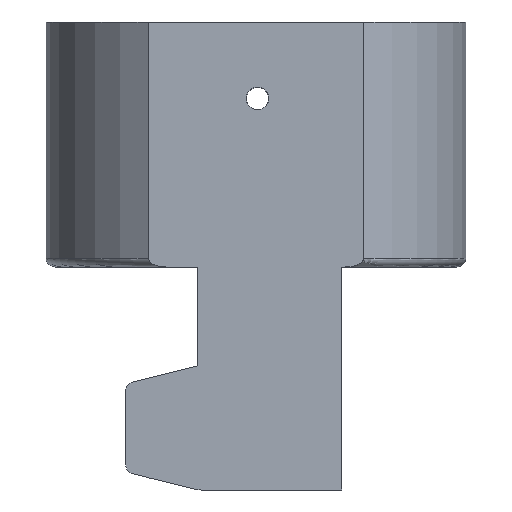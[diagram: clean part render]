
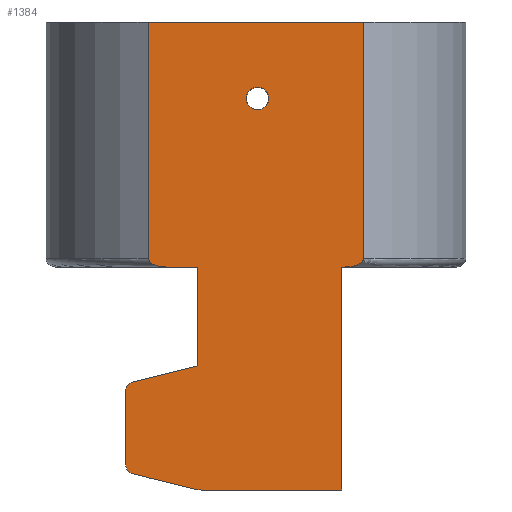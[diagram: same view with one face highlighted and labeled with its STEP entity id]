
A CAD part, front view. The second image highlights one B-rep face of the part: STEP entity #1384.
In plain terms, the highlighted planar face has unit normal (0, -1, 0).
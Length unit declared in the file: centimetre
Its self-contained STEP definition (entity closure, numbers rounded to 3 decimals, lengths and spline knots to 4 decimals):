
#66=FACE_BOUND($,#262,.T.);
#82=PLANE($,#1468);
#96=LINE($,#1725,#133);
#106=LINE($,#1777,#143);
#107=LINE($,#1780,#144);
#109=LINE($,#1786,#146);
#110=LINE($,#1789,#147);
#111=LINE($,#1792,#148);
#114=LINE($,#1802,#151);
#120=LINE($,#1924,#157);
#122=LINE($,#1928,#159);
#123=LINE($,#1932,#160);
#124=LINE($,#1935,#161);
#133=VECTOR($,#1518,2.595);
#143=VECTOR($,#1542,0.339);
#144=VECTOR($,#1545,0.0324);
#146=VECTOR($,#1551,2.3692);
#147=VECTOR($,#1556,2.595);
#148=VECTOR($,#1559,2.4514);
#151=VECTOR($,#1568,1.0861);
#157=VECTOR($,#1604,0.7391);
#159=VECTOR($,#1608,0.8148);
#160=VECTOR($,#1611,0.7025);
#161=VECTOR($,#1614,1.5474);
#199=FACE_OUTER_BOUND($,#261,.T.);
#261=EDGE_LOOP($,(#981,#982,#983,#984,#985,#986,#987,#988,#989,#990,#991,
#992,#993,#994,#995,#996));
#262=EDGE_LOOP($,(#997));
#323=CIRCLE($,#1454,0.099);
#331=CIRCLE($,#1469,0.099);
#332=CIRCLE($,#1470,0.297);
#333=CIRCLE($,#1471,0.1238);
#344=B_SPLINE_CURVE_WITH_KNOTS($,3,(#1707,#1708,#1709,#1710,#1711,#1712,
#1713,#1714,#1715,#1716,#1717,#1718),.UNSPECIFIED.,.F.,.F.,(4,2,2,2,2,4),
(1.0104,1.0239,1.039,1.0807,1.1452,
1.2445),.UNSPECIFIED.);
#346=B_SPLINE_CURVE_WITH_KNOTS($,3,(#1760,#1761,#1762,#1763,#1764,#1765,
#1766,#1767,#1768,#1769,#1770,#1771),.UNSPECIFIED.,.F.,.F.,(4,2,2,2,2,4),
(0.7762,0.8756,0.9401,0.9818,
0.9968,1.0104),.UNSPECIFIED.);
#487=VERTEX_POINT($,#1704);
#488=VERTEX_POINT($,#1706);
#490=VERTEX_POINT($,#1723);
#501=VERTEX_POINT($,#1758);
#502=VERTEX_POINT($,#1759);
#503=VERTEX_POINT($,#1775);
#504=VERTEX_POINT($,#1779);
#506=VERTEX_POINT($,#1785);
#507=VERTEX_POINT($,#1791);
#511=VERTEX_POINT($,#1801);
#512=VERTEX_POINT($,#1805);
#513=VERTEX_POINT($,#1806);
#525=VERTEX_POINT($,#1927);
#526=VERTEX_POINT($,#1929);
#527=VERTEX_POINT($,#1931);
#528=VERTEX_POINT($,#1933);
#529=VERTEX_POINT($,#1936);
#664=EDGE_CURVE($,#487,#488,#344,.T.);
#668=EDGE_CURVE($,#490,#487,#96,.F.);
#680=EDGE_CURVE($,#501,#502,#346,.T.);
#684=EDGE_CURVE($,#503,#501,#106,.T.);
#685=EDGE_CURVE($,#488,#504,#107,.T.);
#688=EDGE_CURVE($,#506,#490,#109,.F.);
#690=EDGE_CURVE($,#502,#506,#110,.F.);
#691=EDGE_CURVE($,#504,#507,#111,.T.);
#696=EDGE_CURVE($,#511,#503,#114,.T.);
#698=EDGE_CURVE($,#512,#513,#323,.T.);
#717=EDGE_CURVE($,#511,#513,#120,.F.);
#719=EDGE_CURVE($,#525,#512,#122,.F.);
#720=EDGE_CURVE($,#526,#525,#331,.T.);
#721=EDGE_CURVE($,#526,#527,#123,.F.);
#722=EDGE_CURVE($,#528,#527,#332,.T.);
#723=EDGE_CURVE($,#507,#528,#124,.F.);
#724=EDGE_CURVE($,#529,#529,#333,.F.);
#981=ORIENTED_EDGE($,*,*,#664,.F.);
#982=ORIENTED_EDGE($,*,*,#668,.F.);
#983=ORIENTED_EDGE($,*,*,#688,.F.);
#984=ORIENTED_EDGE($,*,*,#690,.F.);
#985=ORIENTED_EDGE($,*,*,#680,.F.);
#986=ORIENTED_EDGE($,*,*,#684,.F.);
#987=ORIENTED_EDGE($,*,*,#696,.F.);
#988=ORIENTED_EDGE($,*,*,#717,.T.);
#989=ORIENTED_EDGE($,*,*,#698,.F.);
#990=ORIENTED_EDGE($,*,*,#719,.F.);
#991=ORIENTED_EDGE($,*,*,#720,.F.);
#992=ORIENTED_EDGE($,*,*,#721,.T.);
#993=ORIENTED_EDGE($,*,*,#722,.F.);
#994=ORIENTED_EDGE($,*,*,#723,.F.);
#995=ORIENTED_EDGE($,*,*,#691,.F.);
#996=ORIENTED_EDGE($,*,*,#685,.F.);
#997=ORIENTED_EDGE($,*,*,#724,.F.);
#1384=ADVANCED_FACE($,(#199,#66),#82,.F.);
#1454=AXIS2_PLACEMENT_3D($,#1807,#1572,#1573);
#1468=AXIS2_PLACEMENT_3D($,#1926,#1606,#1607);
#1469=AXIS2_PLACEMENT_3D($,#1930,#1609,#1610);
#1470=AXIS2_PLACEMENT_3D($,#1934,#1612,#1613);
#1471=AXIS2_PLACEMENT_3D($,#1937,#1615,#1616);
#1518=DIRECTION($,(0.,0.,1.));
#1542=DIRECTION($,(-1.,0.,0.));
#1545=DIRECTION($,(-1.,0.,0.));
#1551=DIRECTION($,(-1.,0.,0.));
#1556=DIRECTION($,(0.,0.,-1.));
#1559=DIRECTION($,(0.,0.,-1.));
#1568=DIRECTION($,(0.,0.,1.));
#1572=DIRECTION('center_axis',(0.,1.,0.));
#1573=DIRECTION('ref_axis',(-0.788,0.,0.615));
#1604=DIRECTION($,(0.97,0.,0.243));
#1606=DIRECTION('center_axis',(0.,1.,0.));
#1607=DIRECTION('ref_axis',(-1.,0.,0.));
#1608=DIRECTION($,(0.,0.,-1.));
#1609=DIRECTION('center_axis',(0.,1.,0.));
#1610=DIRECTION('ref_axis',(-0.788,0.,-0.615));
#1611=DIRECTION($,(-0.97,0.,0.243));
#1612=DIRECTION('center_axis',(0.,1.,0.));
#1613=DIRECTION('ref_axis',(-0.122,0.,-0.993));
#1614=DIRECTION($,(1.,0.,0.));
#1615=DIRECTION('center_axis',(0.,1.,0.));
#1616=DIRECTION('ref_axis',(1.,0.,0.));
#1704=CARTESIAN_POINT('',(-9.487,9.0985,4.5504));
#1706=CARTESIAN_POINT('',(-9.6939,9.0985,4.4514));
#1707=CARTESIAN_POINT('Ctrl Pts',(-9.487,9.0985,4.5504));
#1708=CARTESIAN_POINT('Ctrl Pts',(-9.487,9.0985,4.5459));
#1709=CARTESIAN_POINT('Ctrl Pts',(-9.4878,9.0985,4.5406));
#1710=CARTESIAN_POINT('Ctrl Pts',(-9.4904,9.0985,4.5314));
#1711=CARTESIAN_POINT('Ctrl Pts',(-9.4929,9.0985,4.5259));
#1712=CARTESIAN_POINT('Ctrl Pts',(-9.5025,9.0985,4.5097));
#1713=CARTESIAN_POINT('Ctrl Pts',(-9.5149,9.0985,4.4985));
#1714=CARTESIAN_POINT('Ctrl Pts',(-9.5444,9.0985,4.4789));
#1715=CARTESIAN_POINT('Ctrl Pts',(-9.5684,9.0985,4.4696));
#1716=CARTESIAN_POINT('Ctrl Pts',(-9.6212,9.0985,4.4554));
#1717=CARTESIAN_POINT('Ctrl Pts',(-9.6608,9.0985,4.4514));
#1718=CARTESIAN_POINT('Ctrl Pts',(-9.6939,9.0985,4.4514));
#1723=CARTESIAN_POINT('',(-9.487,9.0985,7.1454));
#1725=CARTESIAN_POINT($,(-9.487,9.0985,8.8847));
#1758=CARTESIAN_POINT('',(-11.6493,9.0985,4.4514));
#1759=CARTESIAN_POINT('',(-11.8562,9.0985,4.5504));
#1760=CARTESIAN_POINT('Ctrl Pts',(-11.6493,9.0985,4.4514));
#1761=CARTESIAN_POINT('Ctrl Pts',(-11.6824,9.0985,4.4514));
#1762=CARTESIAN_POINT('Ctrl Pts',(-11.722,9.0985,4.4554));
#1763=CARTESIAN_POINT('Ctrl Pts',(-11.7748,9.0985,4.4696));
#1764=CARTESIAN_POINT('Ctrl Pts',(-11.7988,9.0985,4.4789));
#1765=CARTESIAN_POINT('Ctrl Pts',(-11.8283,9.0985,4.4985));
#1766=CARTESIAN_POINT('Ctrl Pts',(-11.8407,9.0985,4.5097));
#1767=CARTESIAN_POINT('Ctrl Pts',(-11.8504,9.0985,4.5259));
#1768=CARTESIAN_POINT('Ctrl Pts',(-11.8528,9.0985,4.5314));
#1769=CARTESIAN_POINT('Ctrl Pts',(-11.8554,9.0985,4.5406));
#1770=CARTESIAN_POINT('Ctrl Pts',(-11.8562,9.0985,4.5459));
#1771=CARTESIAN_POINT('Ctrl Pts',(-11.8562,9.0985,4.5504));
#1775=CARTESIAN_POINT('',(-11.3103,9.0985,4.4514));
#1777=CARTESIAN_POINT($,(-11.0404,9.0985,4.4514));
#1779=CARTESIAN_POINT('',(-9.7263,9.0985,4.4514));
#1780=CARTESIAN_POINT($,(-11.0404,9.0985,4.4514));
#1785=CARTESIAN_POINT('',(-11.8562,9.0985,7.1454));
#1786=CARTESIAN_POINT($,(-10.4862,9.0985,7.1454));
#1789=CARTESIAN_POINT($,(-11.8562,9.0985,8.8847));
#1791=CARTESIAN_POINT('',(-9.7263,9.0985,2.));
#1792=CARTESIAN_POINT($,(-9.7263,9.0985,2.6435));
#1801=CARTESIAN_POINT('',(-11.3103,9.0985,3.3654));
#1802=CARTESIAN_POINT($,(-11.3103,9.0985,3.2128));
#1805=CARTESIAN_POINT('',(-12.1023,9.0985,3.0901));
#1806=CARTESIAN_POINT('',(-12.0273,9.0985,3.1861));
#1807=CARTESIAN_POINT('Origin',(-12.0033,9.0985,3.0901));
#1924=CARTESIAN_POINT($,(-11.9196,9.0985,3.2131));
#1926=CARTESIAN_POINT('Origin',(-11.4093,9.0985,2.6435));
#1927=CARTESIAN_POINT('',(-12.1023,9.0985,2.2753));
#1928=CARTESIAN_POINT($,(-12.1023,9.0985,2.6435));
#1929=CARTESIAN_POINT('',(-12.0273,9.0985,2.1793));
#1930=CARTESIAN_POINT('Origin',(-12.0033,9.0985,2.2753));
#1931=CARTESIAN_POINT('',(-11.3458,9.0985,2.0089));
#1932=CARTESIAN_POINT($,(-11.9128,9.0985,2.1506));
#1933=CARTESIAN_POINT('',(-11.2737,9.0985,2.));
#1934=CARTESIAN_POINT('Origin',(-11.2737,9.0985,2.297));
#1935=CARTESIAN_POINT($,(-11.4093,9.0985,2.));
#1936=CARTESIAN_POINT('',(-10.7783,9.0985,6.3039));
#1937=CARTESIAN_POINT('Origin',(-10.6545,9.0985,6.3039));
